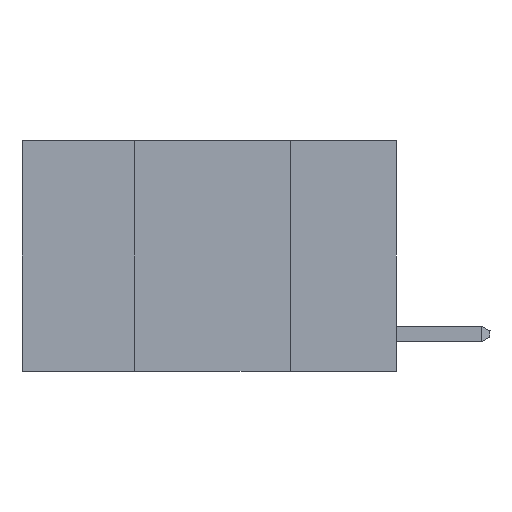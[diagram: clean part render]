
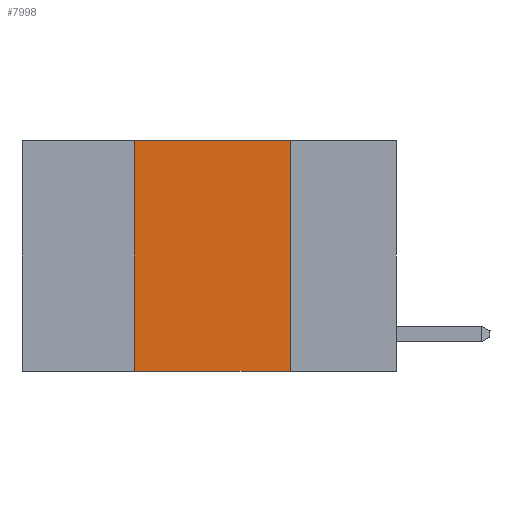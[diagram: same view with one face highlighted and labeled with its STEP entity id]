
A CAD part, left-side view. The second image highlights one B-rep face of the part: STEP entity #7998.
In plain terms, the highlighted planar face has unit normal (-1, 0, 0).
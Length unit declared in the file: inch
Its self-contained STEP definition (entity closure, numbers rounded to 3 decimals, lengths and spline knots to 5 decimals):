
#161 = CARTESIAN_POINT ( 'NONE',  ( 0., 0.6, 0. ) ) ;
#578 = EDGE_LOOP ( 'NONE', ( #1511, #8975, #9472, #7794 ) ) ;
#1010 = EDGE_CURVE ( 'NONE', #6859, #7807, #5966, .T. ) ;
#1511 = ORIENTED_EDGE ( 'NONE', *, *, #5350, .F. ) ;
#1666 = CARTESIAN_POINT ( 'NONE',  ( 0., 0.6, -0.37 ) ) ;
#1789 = VECTOR ( 'NONE', #6713, 39.37008 ) ;
#1961 = VERTEX_POINT ( 'NONE', #6592 ) ;
#2758 = LINE ( 'NONE', #5158, #1789 ) ;
#3099 = FACE_OUTER_BOUND ( 'NONE', #578, .T. ) ;
#3406 = DIRECTION ( 'NONE',  ( 0., 0., -1. ) ) ;
#3513 = AXIS2_PLACEMENT_3D ( 'NONE', #8577, #6622, #3406 ) ;
#3640 = DIRECTION ( 'NONE',  ( 0., -1., 0. ) ) ;
#4443 = VECTOR ( 'NONE', #8796, 39.37008 ) ;
#4525 = CARTESIAN_POINT ( 'NONE',  ( 0., 0.42, -0.37 ) ) ;
#5123 = EDGE_CURVE ( 'NONE', #7807, #1961, #5526, .T. ) ;
#5158 = CARTESIAN_POINT ( 'NONE',  ( 0., 0.17, 0. ) ) ;
#5350 = EDGE_CURVE ( 'NONE', #1961, #10653, #2758, .T. ) ;
#5526 = LINE ( 'NONE', #161, #10187 ) ;
#5819 = CARTESIAN_POINT ( 'NONE',  ( 0., 0.42, 0. ) ) ;
#5966 = LINE ( 'NONE', #5819, #9301 ) ;
#5992 = CARTESIAN_POINT ( 'NONE',  ( 0., 0.42, 0. ) ) ;
#6188 = LINE ( 'NONE', #1666, #4443 ) ;
#6592 = CARTESIAN_POINT ( 'NONE',  ( 0., 0.17, 0. ) ) ;
#6622 = DIRECTION ( 'NONE',  ( 1., 0., 0. ) ) ;
#6713 = DIRECTION ( 'NONE',  ( 0., 0., -1. ) ) ;
#6859 = VERTEX_POINT ( 'NONE', #4525 ) ;
#7684 = PLANE ( 'NONE',  #3513 ) ;
#7794 = ORIENTED_EDGE ( 'NONE', *, *, #9037, .T. ) ;
#7807 = VERTEX_POINT ( 'NONE', #5992 ) ;
#7998 = ADVANCED_FACE ( 'NONE', ( #3099 ), #7684, .F. ) ;
#8577 = CARTESIAN_POINT ( 'NONE',  ( 0., 0.6, 0. ) ) ;
#8796 = DIRECTION ( 'NONE',  ( 0., -1., 0. ) ) ;
#8975 = ORIENTED_EDGE ( 'NONE', *, *, #5123, .F. ) ;
#9037 = EDGE_CURVE ( 'NONE', #6859, #10653, #6188, .T. ) ;
#9301 = VECTOR ( 'NONE', #11099, 39.37008 ) ;
#9472 = ORIENTED_EDGE ( 'NONE', *, *, #1010, .F. ) ;
#10187 = VECTOR ( 'NONE', #3640, 39.37008 ) ;
#10653 = VERTEX_POINT ( 'NONE', #11054 ) ;
#11054 = CARTESIAN_POINT ( 'NONE',  ( 0., 0.17, -0.37 ) ) ;
#11099 = DIRECTION ( 'NONE',  ( 0., 0., 1. ) ) ;
